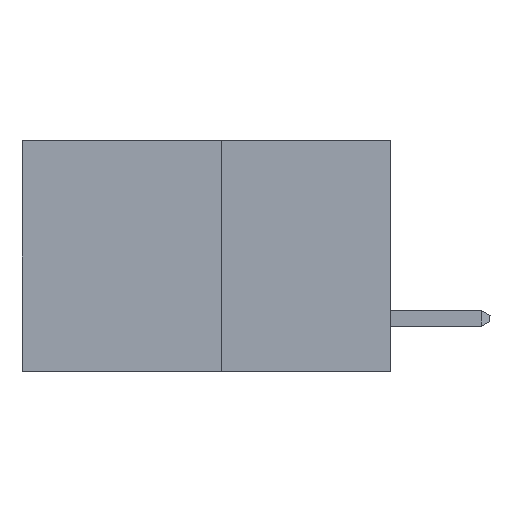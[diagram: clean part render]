
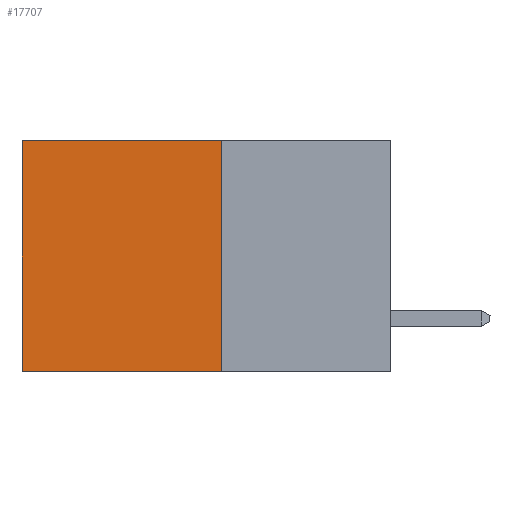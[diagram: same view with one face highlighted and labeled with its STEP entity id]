
A CAD part, left-side view. The second image highlights one B-rep face of the part: STEP entity #17707.
In plain terms, the highlighted planar face has unit normal (-1, 0, 0).
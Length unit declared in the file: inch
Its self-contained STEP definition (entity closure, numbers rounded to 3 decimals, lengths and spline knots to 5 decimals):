
#596 = VERTEX_POINT ( 'NONE', #21362 ) ;
#966 = VECTOR ( 'NONE', #17955, 39.37008 ) ;
#1461 = EDGE_CURVE ( 'NONE', #10558, #596, #8616, .T. ) ;
#1514 = DIRECTION ( 'NONE',  ( 0., 0., -1. ) ) ;
#1643 = DIRECTION ( 'NONE',  ( 1., 0., 0. ) ) ;
#2115 = ORIENTED_EDGE ( 'NONE', *, *, #24967, .F. ) ;
#3030 = ORIENTED_EDGE ( 'NONE', *, *, #27607, .F. ) ;
#3481 = CARTESIAN_POINT ( 'NONE',  ( 0.277, 0.27, -0.37 ) ) ;
#4129 = VECTOR ( 'NONE', #10810, 39.37008 ) ;
#4895 = LINE ( 'NONE', #3481, #4129 ) ;
#5905 = VECTOR ( 'NONE', #26876, 39.37008 ) ;
#8616 = LINE ( 'NONE', #11531, #21328 ) ;
#9288 = ORIENTED_EDGE ( 'NONE', *, *, #26732, .T. ) ;
#10041 = CARTESIAN_POINT ( 'NONE',  ( 0.277, 0.27, 0. ) ) ;
#10558 = VERTEX_POINT ( 'NONE', #23467 ) ;
#10810 = DIRECTION ( 'NONE',  ( 0., 0., -1. ) ) ;
#11531 = CARTESIAN_POINT ( 'NONE',  ( 0.277, 0.59, -0.37 ) ) ;
#12362 = LINE ( 'NONE', #22110, #5905 ) ;
#15591 = CARTESIAN_POINT ( 'NONE',  ( 0.277, 0.27, -0.37 ) ) ;
#16091 = CARTESIAN_POINT ( 'NONE',  ( 0.277, 0.27, -0.37 ) ) ;
#16348 = AXIS2_PLACEMENT_3D ( 'NONE', #16091, #1643, #18476 ) ;
#17707 = ADVANCED_FACE ( 'NONE', ( #27806 ), #23173, .F. ) ;
#17955 = DIRECTION ( 'NONE',  ( 0., 1., 0. ) ) ;
#18476 = DIRECTION ( 'NONE',  ( 0., 0., -1. ) ) ;
#18696 = ORIENTED_EDGE ( 'NONE', *, *, #1461, .T. ) ;
#19386 = LINE ( 'NONE', #15591, #966 ) ;
#21328 = VECTOR ( 'NONE', #1514, 39.37008 ) ;
#21362 = CARTESIAN_POINT ( 'NONE',  ( 0.277, 0.59, -0.37 ) ) ;
#22110 = CARTESIAN_POINT ( 'NONE',  ( 0.277, 0.27, 0. ) ) ;
#23173 = PLANE ( 'NONE',  #16348 ) ;
#23467 = CARTESIAN_POINT ( 'NONE',  ( 0.277, 0.59, 0. ) ) ;
#24967 = EDGE_CURVE ( 'NONE', #29304, #30326, #4895, .T. ) ;
#26060 = CARTESIAN_POINT ( 'NONE',  ( 0.277, 0.27, -0.37 ) ) ;
#26732 = EDGE_CURVE ( 'NONE', #29304, #10558, #12362, .T. ) ;
#26876 = DIRECTION ( 'NONE',  ( 0., 1., 0. ) ) ;
#27607 = EDGE_CURVE ( 'NONE', #30326, #596, #19386, .T. ) ;
#27806 = FACE_OUTER_BOUND ( 'NONE', #29601, .T. ) ;
#29304 = VERTEX_POINT ( 'NONE', #10041 ) ;
#29601 = EDGE_LOOP ( 'NONE', ( #18696, #3030, #2115, #9288 ) ) ;
#30326 = VERTEX_POINT ( 'NONE', #26060 ) ;
